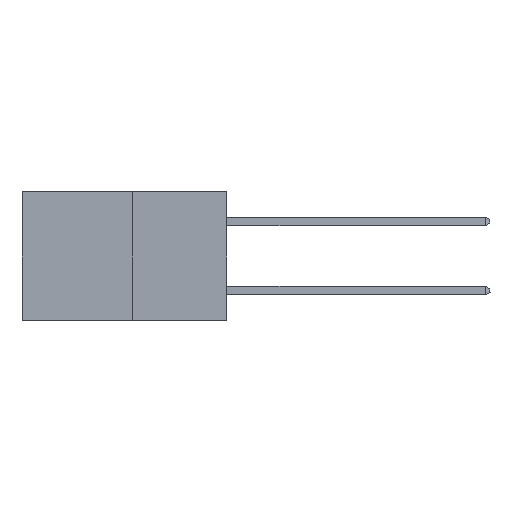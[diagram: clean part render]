
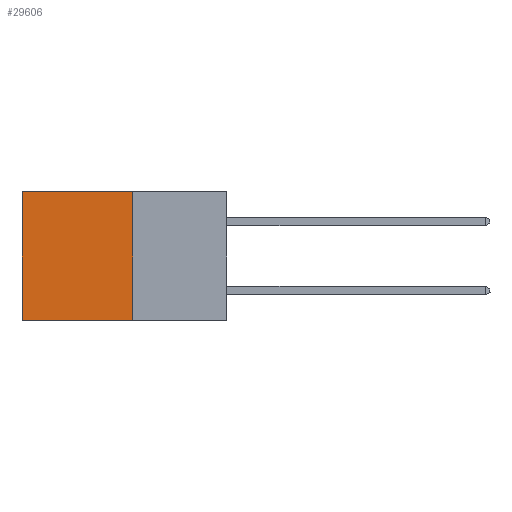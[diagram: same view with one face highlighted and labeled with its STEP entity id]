
A CAD part, left-side view. The second image highlights one B-rep face of the part: STEP entity #29606.
In plain terms, the highlighted planar face has unit normal (-1, 0, 0).
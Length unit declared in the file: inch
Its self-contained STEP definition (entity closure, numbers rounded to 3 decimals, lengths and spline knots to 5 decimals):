
#676 = DIRECTION ( 'NONE',  ( 0., 0., -1. ) ) ;
#902 = CARTESIAN_POINT ( 'NONE',  ( 0.277, 0.59, -0.37 ) ) ;
#1140 = ORIENTED_EDGE ( 'NONE', *, *, #28438, .F. ) ;
#1217 = EDGE_CURVE ( 'NONE', #27896, #7814, #29367, .T. ) ;
#2350 = FACE_OUTER_BOUND ( 'NONE', #5529, .T. ) ;
#3327 = AXIS2_PLACEMENT_3D ( 'NONE', #19172, #14636, #676 ) ;
#5529 = EDGE_LOOP ( 'NONE', ( #9200, #13175, #1140, #25016 ) ) ;
#7189 = CARTESIAN_POINT ( 'NONE',  ( 0.277, 0.59, 0. ) ) ;
#7305 = VERTEX_POINT ( 'NONE', #27059 ) ;
#7494 = DIRECTION ( 'NONE',  ( 0., 0., -1. ) ) ;
#7559 = CARTESIAN_POINT ( 'NONE',  ( 0.277, 0.59, -0.37 ) ) ;
#7814 = VERTEX_POINT ( 'NONE', #902 ) ;
#9200 = ORIENTED_EDGE ( 'NONE', *, *, #1217, .T. ) ;
#10045 = VECTOR ( 'NONE', #28205, 39.37008 ) ;
#11004 = VECTOR ( 'NONE', #7494, 39.37008 ) ;
#12612 = CARTESIAN_POINT ( 'NONE',  ( 0.277, 0.27, -0.37 ) ) ;
#13175 = ORIENTED_EDGE ( 'NONE', *, *, #23198, .F. ) ;
#13486 = LINE ( 'NONE', #12612, #25736 ) ;
#14636 = DIRECTION ( 'NONE',  ( 1., 0., 0. ) ) ;
#14926 = DIRECTION ( 'NONE',  ( 0., 1., 0. ) ) ;
#15876 = CARTESIAN_POINT ( 'NONE',  ( 0.277, 0.27, -0.37 ) ) ;
#19012 = CARTESIAN_POINT ( 'NONE',  ( 0.277, 0.27, -0.37 ) ) ;
#19172 = CARTESIAN_POINT ( 'NONE',  ( 0.277, 0.27, -0.37 ) ) ;
#19346 = VERTEX_POINT ( 'NONE', #19012 ) ;
#20529 = DIRECTION ( 'NONE',  ( 0., 0., -1. ) ) ;
#22044 = VECTOR ( 'NONE', #20529, 39.37008 ) ;
#23198 = EDGE_CURVE ( 'NONE', #19346, #7814, #13486, .T. ) ;
#25016 = ORIENTED_EDGE ( 'NONE', *, *, #29534, .T. ) ;
#25736 = VECTOR ( 'NONE', #14926, 39.37008 ) ;
#27059 = CARTESIAN_POINT ( 'NONE',  ( 0.277, 0.27, 0. ) ) ;
#27896 = VERTEX_POINT ( 'NONE', #7189 ) ;
#28106 = CARTESIAN_POINT ( 'NONE',  ( 0.277, 0.27, 0. ) ) ;
#28124 = LINE ( 'NONE', #15876, #22044 ) ;
#28205 = DIRECTION ( 'NONE',  ( 0., 1., 0. ) ) ;
#28404 = PLANE ( 'NONE',  #3327 ) ;
#28413 = LINE ( 'NONE', #28106, #10045 ) ;
#28438 = EDGE_CURVE ( 'NONE', #7305, #19346, #28124, .T. ) ;
#29367 = LINE ( 'NONE', #7559, #11004 ) ;
#29534 = EDGE_CURVE ( 'NONE', #7305, #27896, #28413, .T. ) ;
#29606 = ADVANCED_FACE ( 'NONE', ( #2350 ), #28404, .F. ) ;
